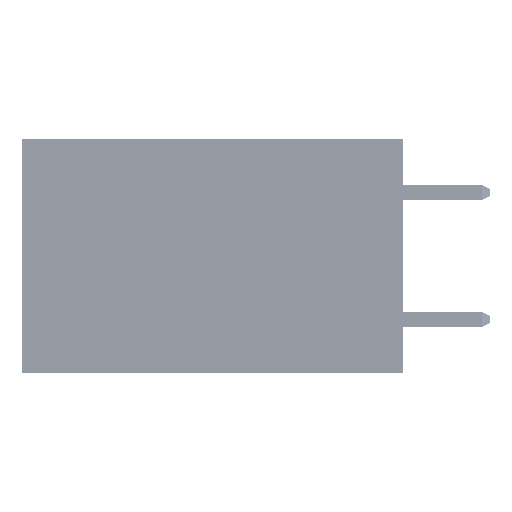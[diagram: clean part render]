
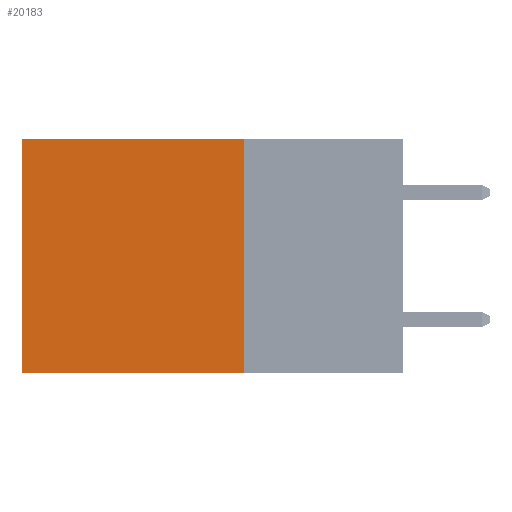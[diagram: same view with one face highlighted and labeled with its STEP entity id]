
A CAD part, left-side view. The second image highlights one B-rep face of the part: STEP entity #20183.
In plain terms, the highlighted planar face has unit normal (-1, 0, 0).
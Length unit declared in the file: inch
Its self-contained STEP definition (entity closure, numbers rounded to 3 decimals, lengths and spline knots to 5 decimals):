
#827 = LINE ( 'NONE', #21244, #28427 ) ;
#1006 = VECTOR ( 'NONE', #52920, 39.37008 ) ;
#2202 = DIRECTION ( 'NONE',  ( 0., 0., -1. ) ) ;
#3757 = ORIENTED_EDGE ( 'NONE', *, *, #38407, .F. ) ;
#7056 = FACE_OUTER_BOUND ( 'NONE', #29699, .T. ) ;
#7592 = VERTEX_POINT ( 'NONE', #47536 ) ;
#8049 = LINE ( 'NONE', #48799, #1006 ) ;
#10099 = DIRECTION ( 'NONE',  ( 0., 0., -1. ) ) ;
#11862 = CARTESIAN_POINT ( 'NONE',  ( 0.2875, 0.25, -0.37 ) ) ;
#18488 = CARTESIAN_POINT ( 'NONE',  ( 0.2875, 0.25, 0. ) ) ;
#20183 = ADVANCED_FACE ( 'NONE', ( #7056 ), #30389, .F. ) ;
#21244 = CARTESIAN_POINT ( 'NONE',  ( 0.2875, 0.6, 0. ) ) ;
#22628 = EDGE_CURVE ( 'NONE', #7592, #44756, #8049, .T. ) ;
#26590 = ORIENTED_EDGE ( 'NONE', *, *, #27478, .T. ) ;
#27478 = EDGE_CURVE ( 'NONE', #44756, #36074, #827, .T. ) ;
#27927 = VERTEX_POINT ( 'NONE', #11862 ) ;
#28427 = VECTOR ( 'NONE', #45433, 39.37008 ) ;
#29295 = AXIS2_PLACEMENT_3D ( 'NONE', #51445, #34676, #10099 ) ;
#29699 = EDGE_LOOP ( 'NONE', ( #26590, #50577, #3757, #46850 ) ) ;
#30389 = PLANE ( 'NONE',  #29295 ) ;
#34676 = DIRECTION ( 'NONE',  ( 1., 0., 0. ) ) ;
#36074 = VERTEX_POINT ( 'NONE', #52620 ) ;
#37600 = LINE ( 'NONE', #42351, #48494 ) ;
#38258 = DIRECTION ( 'NONE',  ( 0., 1., 0. ) ) ;
#38407 = EDGE_CURVE ( 'NONE', #7592, #27927, #40300, .T. ) ;
#40300 = LINE ( 'NONE', #18488, #52477 ) ;
#42351 = CARTESIAN_POINT ( 'NONE',  ( 0.2875, 0.25, -0.37 ) ) ;
#44756 = VERTEX_POINT ( 'NONE', #52982 ) ;
#45433 = DIRECTION ( 'NONE',  ( 0., 0., -1. ) ) ;
#46850 = ORIENTED_EDGE ( 'NONE', *, *, #22628, .T. ) ;
#47536 = CARTESIAN_POINT ( 'NONE',  ( 0.2875, 0.25, 0. ) ) ;
#48111 = EDGE_CURVE ( 'NONE', #27927, #36074, #37600, .T. ) ;
#48494 = VECTOR ( 'NONE', #38258, 39.37008 ) ;
#48799 = CARTESIAN_POINT ( 'NONE',  ( 0.2875, 0.25, 0. ) ) ;
#50577 = ORIENTED_EDGE ( 'NONE', *, *, #48111, .F. ) ;
#51445 = CARTESIAN_POINT ( 'NONE',  ( 0.2875, 0.25, 0. ) ) ;
#52477 = VECTOR ( 'NONE', #2202, 39.37008 ) ;
#52620 = CARTESIAN_POINT ( 'NONE',  ( 0.2875, 0.6, -0.37 ) ) ;
#52920 = DIRECTION ( 'NONE',  ( 0., 1., 0. ) ) ;
#52982 = CARTESIAN_POINT ( 'NONE',  ( 0.2875, 0.6, 0. ) ) ;
